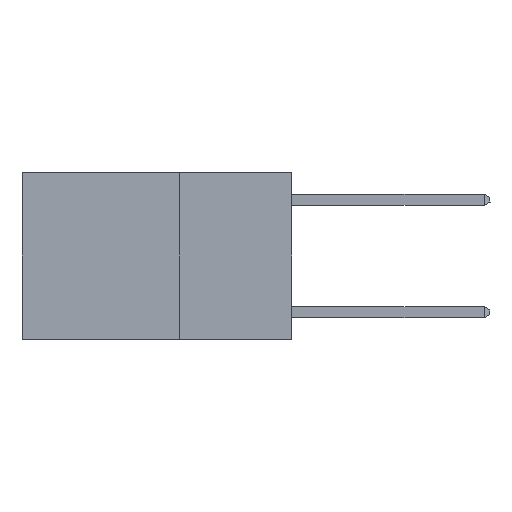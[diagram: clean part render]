
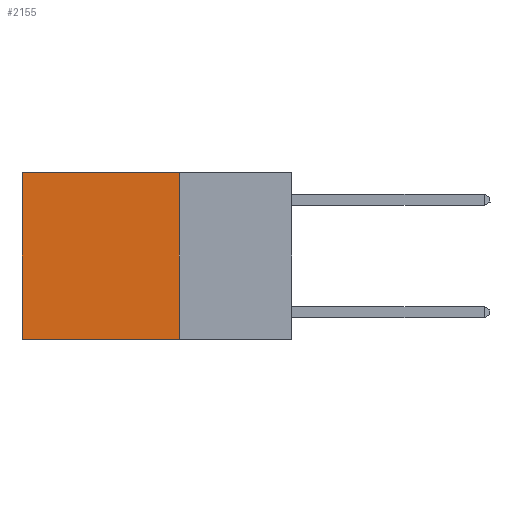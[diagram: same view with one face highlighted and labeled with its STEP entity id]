
A CAD part, left-side view. The second image highlights one B-rep face of the part: STEP entity #2155.
In plain terms, the highlighted planar face has unit normal (-1, 0, 0).
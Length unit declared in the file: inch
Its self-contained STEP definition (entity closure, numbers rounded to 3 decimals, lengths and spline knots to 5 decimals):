
#90 = DIRECTION ( 'NONE',  ( 0., 0., -1. ) ) ;
#731 = LINE ( 'NONE', #4238, #13691 ) ;
#751 = CARTESIAN_POINT ( 'NONE',  ( 0.2625, 0.25, -0.37 ) ) ;
#2155 = ADVANCED_FACE ( 'NONE', ( #8732 ), #8233, .F. ) ;
#2959 = LINE ( 'NONE', #13662, #10223 ) ;
#3747 = VERTEX_POINT ( 'NONE', #8397 ) ;
#4028 = EDGE_CURVE ( 'NONE', #4377, #10903, #2959, .T. ) ;
#4238 = CARTESIAN_POINT ( 'NONE',  ( 0.2625, 0.25, 0. ) ) ;
#4377 = VERTEX_POINT ( 'NONE', #751 ) ;
#4964 = CARTESIAN_POINT ( 'NONE',  ( 0.2625, 0.25, 0. ) ) ;
#5872 = CARTESIAN_POINT ( 'NONE',  ( 0.2625, 0.6, -0.37 ) ) ;
#6287 = DIRECTION ( 'NONE',  ( 0., 0., -1. ) ) ;
#6498 = DIRECTION ( 'NONE',  ( 0., 1., 0. ) ) ;
#7067 = DIRECTION ( 'NONE',  ( 0., 0., -1. ) ) ;
#7073 = EDGE_CURVE ( 'NONE', #13776, #10903, #7224, .T. ) ;
#7115 = AXIS2_PLACEMENT_3D ( 'NONE', #15281, #14145, #7067 ) ;
#7224 = LINE ( 'NONE', #13880, #13205 ) ;
#8233 = PLANE ( 'NONE',  #7115 ) ;
#8397 = CARTESIAN_POINT ( 'NONE',  ( 0.2625, 0.25, 0. ) ) ;
#8616 = CARTESIAN_POINT ( 'NONE',  ( 0.2625, 0.6, 0. ) ) ;
#8711 = LINE ( 'NONE', #4964, #14520 ) ;
#8732 = FACE_OUTER_BOUND ( 'NONE', #13080, .T. ) ;
#9403 = DIRECTION ( 'NONE',  ( 0., 1., 0. ) ) ;
#9524 = EDGE_CURVE ( 'NONE', #3747, #13776, #731, .T. ) ;
#10223 = VECTOR ( 'NONE', #6498, 39.37008 ) ;
#10224 = EDGE_CURVE ( 'NONE', #3747, #4377, #8711, .T. ) ;
#10903 = VERTEX_POINT ( 'NONE', #5872 ) ;
#13080 = EDGE_LOOP ( 'NONE', ( #13569, #13624, #13626, #14299 ) ) ;
#13205 = VECTOR ( 'NONE', #90, 39.37008 ) ;
#13569 = ORIENTED_EDGE ( 'NONE', *, *, #7073, .T. ) ;
#13624 = ORIENTED_EDGE ( 'NONE', *, *, #4028, .F. ) ;
#13626 = ORIENTED_EDGE ( 'NONE', *, *, #10224, .F. ) ;
#13662 = CARTESIAN_POINT ( 'NONE',  ( 0.2625, 0.25, -0.37 ) ) ;
#13691 = VECTOR ( 'NONE', #9403, 39.37008 ) ;
#13776 = VERTEX_POINT ( 'NONE', #8616 ) ;
#13880 = CARTESIAN_POINT ( 'NONE',  ( 0.2625, 0.6, 0. ) ) ;
#14145 = DIRECTION ( 'NONE',  ( 1., 0., 0. ) ) ;
#14299 = ORIENTED_EDGE ( 'NONE', *, *, #9524, .T. ) ;
#14520 = VECTOR ( 'NONE', #6287, 39.37008 ) ;
#15281 = CARTESIAN_POINT ( 'NONE',  ( 0.2625, 0.25, 0. ) ) ;
